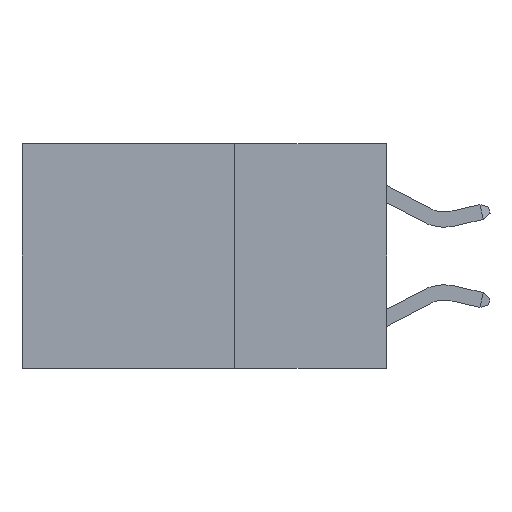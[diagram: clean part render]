
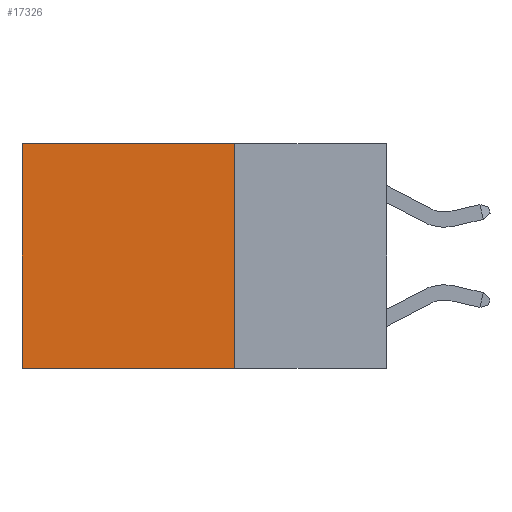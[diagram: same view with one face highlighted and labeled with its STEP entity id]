
A CAD part, left-side view. The second image highlights one B-rep face of the part: STEP entity #17326.
In plain terms, the highlighted planar face has unit normal (-1, 0, 0).
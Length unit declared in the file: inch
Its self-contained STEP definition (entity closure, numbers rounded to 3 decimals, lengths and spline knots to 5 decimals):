
#271 = VERTEX_POINT ( 'NONE', #2515 ) ;
#558 = AXIS2_PLACEMENT_3D ( 'NONE', #2007, #13226, #16117 ) ;
#733 = CARTESIAN_POINT ( 'NONE',  ( 0.2625, 0.25, 0. ) ) ;
#825 = LINE ( 'NONE', #733, #11405 ) ;
#1241 = EDGE_CURVE ( 'NONE', #9042, #2491, #16348, .T. ) ;
#2007 = CARTESIAN_POINT ( 'NONE',  ( 0.2625, 0.25, 0. ) ) ;
#2195 = DIRECTION ( 'NONE',  ( 0., 0., -1. ) ) ;
#2406 = CARTESIAN_POINT ( 'NONE',  ( 0.2625, 0.25, 0. ) ) ;
#2439 = DIRECTION ( 'NONE',  ( 0., 1., 0. ) ) ;
#2491 = VERTEX_POINT ( 'NONE', #17306 ) ;
#2515 = CARTESIAN_POINT ( 'NONE',  ( 0.2625, 0.25, -0.37 ) ) ;
#3529 = EDGE_CURVE ( 'NONE', #271, #4083, #15173, .T. ) ;
#3613 = DIRECTION ( 'NONE',  ( 0., 1., 0. ) ) ;
#4044 = EDGE_CURVE ( 'NONE', #9042, #271, #825, .T. ) ;
#4083 = VERTEX_POINT ( 'NONE', #16788 ) ;
#5479 = VECTOR ( 'NONE', #8770, 39.37008 ) ;
#5966 = ORIENTED_EDGE ( 'NONE', *, *, #1241, .T. ) ;
#6020 = PLANE ( 'NONE',  #558 ) ;
#7581 = EDGE_CURVE ( 'NONE', #2491, #4083, #10528, .T. ) ;
#7593 = CARTESIAN_POINT ( 'NONE',  ( 0.2625, 0.6, 0. ) ) ;
#8770 = DIRECTION ( 'NONE',  ( 0., 0., -1. ) ) ;
#9042 = VERTEX_POINT ( 'NONE', #2406 ) ;
#10528 = LINE ( 'NONE', #7593, #5479 ) ;
#11405 = VECTOR ( 'NONE', #2195, 39.37008 ) ;
#11416 = ORIENTED_EDGE ( 'NONE', *, *, #4044, .F. ) ;
#11583 = ORIENTED_EDGE ( 'NONE', *, *, #7581, .T. ) ;
#13226 = DIRECTION ( 'NONE',  ( 1., 0., 0. ) ) ;
#13445 = CARTESIAN_POINT ( 'NONE',  ( 0.2625, 0.25, 0. ) ) ;
#14373 = VECTOR ( 'NONE', #2439, 39.37008 ) ;
#15127 = ORIENTED_EDGE ( 'NONE', *, *, #3529, .F. ) ;
#15173 = LINE ( 'NONE', #15449, #14373 ) ;
#15449 = CARTESIAN_POINT ( 'NONE',  ( 0.2625, 0.25, -0.37 ) ) ;
#15673 = VECTOR ( 'NONE', #3613, 39.37008 ) ;
#15940 = FACE_OUTER_BOUND ( 'NONE', #17476, .T. ) ;
#16117 = DIRECTION ( 'NONE',  ( 0., 0., -1. ) ) ;
#16348 = LINE ( 'NONE', #13445, #15673 ) ;
#16788 = CARTESIAN_POINT ( 'NONE',  ( 0.2625, 0.6, -0.37 ) ) ;
#17306 = CARTESIAN_POINT ( 'NONE',  ( 0.2625, 0.6, 0. ) ) ;
#17326 = ADVANCED_FACE ( 'NONE', ( #15940 ), #6020, .F. ) ;
#17476 = EDGE_LOOP ( 'NONE', ( #11583, #15127, #11416, #5966 ) ) ;
